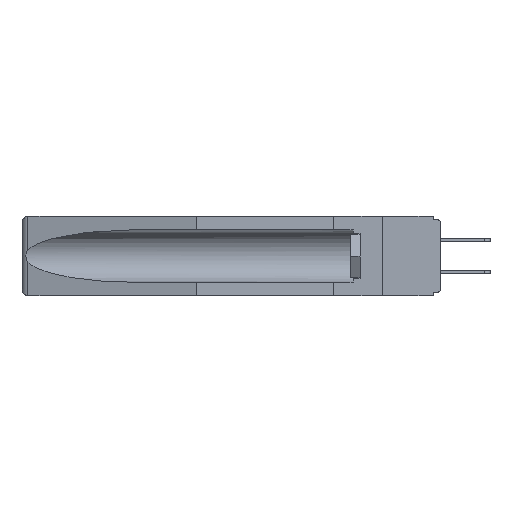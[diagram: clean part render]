
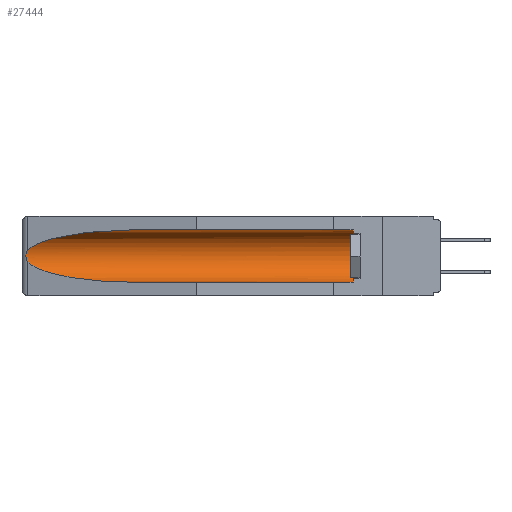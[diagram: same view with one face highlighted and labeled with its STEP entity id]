
A CAD part, left-side view. The second image highlights one B-rep face of the part: STEP entity #27444.
In plain terms, the highlighted cylindrical face has radius 2.857 mm (diameter 5.715 mm), a partial arc.
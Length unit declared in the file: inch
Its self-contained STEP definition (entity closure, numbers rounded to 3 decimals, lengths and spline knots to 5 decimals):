
#496 = CARTESIAN_POINT ( 'NONE',  ( 0.155, 1.07973, -0.059 ) ) ;
#643 = ORIENTED_EDGE ( 'NONE', *, *, #29345, .T. ) ;
#937 = CARTESIAN_POINT ( 'NONE',  ( 0.155, 1.07973, -0.284 ) ) ;
#1045 = CARTESIAN_POINT ( 'NONE',  ( 0.2675, 1.53308, -0.17534 ) ) ;
#1240 = CARTESIAN_POINT ( 'NONE',  ( 0.21114, 1.30732, -0.284 ) ) ;
#2816 = ORIENTED_EDGE ( 'NONE', *, *, #14359, .T. ) ;
#3269 = LINE ( 'NONE', #20191, #4945 ) ;
#3373 =( BOUNDED_CURVE ( )  B_SPLINE_CURVE ( 3, ( #26966, #29349, #1240, #937 ),
 .UNSPECIFIED., .F., .F. ) 
 B_SPLINE_CURVE_WITH_KNOTS ( ( 4, 4 ),
 ( 0.1948, 1.5708 ),
 .UNSPECIFIED. ) 
 CURVE ( )  GEOMETRIC_REPRESENTATION_ITEM ( )  RATIONAL_B_SPLINE_CURVE ( ( 1., 0.848, 0.848, 1. ) ) 
 REPRESENTATION_ITEM ( '' )  );
#3856 = DIRECTION ( 'NONE',  ( 0., 1., 0. ) ) ;
#4360 = CARTESIAN_POINT ( 'NONE',  ( 0.155, 0.126, -0.284 ) ) ;
#4464 = VERTEX_POINT ( 'NONE', #4360 ) ;
#4945 = VECTOR ( 'NONE', #3856, 39.37008 ) ;
#5256 = B_SPLINE_CURVE_WITH_KNOTS ( 'NONE', 3,
 ( #29054, #17379, #21716, #12756, #12349, #1045, #10107, #22134, #5476, #19750 ),
 .UNSPECIFIED., .F., .F.,
 ( 4, 2, 2, 2, 4 ),
 ( 0., 0.00029, 0.00058, 0.00087, 0.00117 ),
 .UNSPECIFIED. ) ;
#5476 = CARTESIAN_POINT ( 'NONE',  ( 0.26597, 1.5296, -0.19026 ) ) ;
#5638 = ORIENTED_EDGE ( 'NONE', *, *, #29744, .T. ) ;
#6762 = CARTESIAN_POINT ( 'NONE',  ( 0.155, 1.07973, -0.284 ) ) ;
#7711 = FACE_OUTER_BOUND ( 'NONE', #21540, .T. ) ;
#7997 = CARTESIAN_POINT ( 'NONE',  ( 0.155, 1.07973, -0.059 ) ) ;
#8139 = DIRECTION ( 'NONE',  ( 0., 1., 0. ) ) ;
#8289 = CARTESIAN_POINT ( 'NONE',  ( 0.26537, 1.52718, -0.14972 ) ) ;
#8427 = VECTOR ( 'NONE', #8139, 39.37008 ) ;
#10078 = DIRECTION ( 'NONE',  ( 0., 0., 1. ) ) ;
#10107 = CARTESIAN_POINT ( 'NONE',  ( 0.2673, 1.53269, -0.17917 ) ) ;
#10977 = CYLINDRICAL_SURFACE ( 'NONE', #28763, 0.1125 ) ;
#12308 = EDGE_CURVE ( 'NONE', #12844, #26190, #5256, .T. ) ;
#12349 = CARTESIAN_POINT ( 'NONE',  ( 0.2675, 1.53308, -0.16763 ) ) ;
#12756 = CARTESIAN_POINT ( 'NONE',  ( 0.2673, 1.5327, -0.16383 ) ) ;
#12844 = VERTEX_POINT ( 'NONE', #15924 ) ;
#13463 = DIRECTION ( 'NONE',  ( 0., -1., 0. ) ) ;
#14108 = CIRCLE ( 'NONE', #27047, 0.1125 ) ;
#14334 = VERTEX_POINT ( 'NONE', #17928 ) ;
#14359 = EDGE_CURVE ( 'NONE', #14334, #29452, #3269, .T. ) ;
#14971 = CARTESIAN_POINT ( 'NONE',  ( 0.155, -0.30754, -0.284 ) ) ;
#15711 = EDGE_CURVE ( 'NONE', #4464, #17910, #28707, .T. ) ;
#15924 = CARTESIAN_POINT ( 'NONE',  ( 0.26537, 1.52718, -0.14972 ) ) ;
#17042 = DIRECTION ( 'NONE',  ( 0., 1., 0. ) ) ;
#17379 = CARTESIAN_POINT ( 'NONE',  ( 0.26597, 1.52961, -0.15275 ) ) ;
#17608 = CARTESIAN_POINT ( 'NONE',  ( 0.25451, 1.48313, -0.09465 ) ) ;
#17910 = VERTEX_POINT ( 'NONE', #6762 ) ;
#17928 = CARTESIAN_POINT ( 'NONE',  ( 0.155, 0.126, -0.059 ) ) ;
#18120 = DIRECTION ( 'NONE',  ( 0., 0., 1. ) ) ;
#18223 = CARTESIAN_POINT ( 'NONE',  ( 0.155, 0.126, -0.1715 ) ) ;
#19185 = ORIENTED_EDGE ( 'NONE', *, *, #15711, .F. ) ;
#19750 = CARTESIAN_POINT ( 'NONE',  ( 0.26537, 1.52718, -0.19328 ) ) ;
#20191 = CARTESIAN_POINT ( 'NONE',  ( 0.155, -0.30754, -0.059 ) ) ;
#21540 = EDGE_LOOP ( 'NONE', ( #29189, #26014, #643, #19185, #5638, #2816 ) ) ;
#21716 = CARTESIAN_POINT ( 'NONE',  ( 0.26654, 1.53092, -0.15636 ) ) ;
#22134 = CARTESIAN_POINT ( 'NONE',  ( 0.26655, 1.53094, -0.18657 ) ) ;
#22245 = CARTESIAN_POINT ( 'NONE',  ( 0.26537, 1.52718, -0.19328 ) ) ;
#24445 = CARTESIAN_POINT ( 'NONE',  ( 0.21114, 1.30732, -0.059 ) ) ;
#24864 =( BOUNDED_CURVE ( )  B_SPLINE_CURVE ( 3, ( #7997, #24445, #17608, #8289 ),
 .UNSPECIFIED., .F., .F. ) 
 B_SPLINE_CURVE_WITH_KNOTS ( ( 4, 4 ),
 ( 4.71239, 6.08839 ),
 .UNSPECIFIED. ) 
 CURVE ( )  GEOMETRIC_REPRESENTATION_ITEM ( )  RATIONAL_B_SPLINE_CURVE ( ( 1., 0.848, 0.848, 1. ) ) 
 REPRESENTATION_ITEM ( '' )  );
#26014 = ORIENTED_EDGE ( 'NONE', *, *, #12308, .T. ) ;
#26190 = VERTEX_POINT ( 'NONE', #22245 ) ;
#26966 = CARTESIAN_POINT ( 'NONE',  ( 0.26537, 1.52718, -0.19328 ) ) ;
#27047 = AXIS2_PLACEMENT_3D ( 'NONE', #18223, #13463, #18120 ) ;
#27444 = ADVANCED_FACE ( 'NONE', ( #7711 ), #10977, .F. ) ;
#27722 = EDGE_CURVE ( 'NONE', #29452, #12844, #24864, .T. ) ;
#28707 = LINE ( 'NONE', #14971, #8427 ) ;
#28763 = AXIS2_PLACEMENT_3D ( 'NONE', #29243, #17042, #10078 ) ;
#29054 = CARTESIAN_POINT ( 'NONE',  ( 0.26537, 1.52718, -0.14972 ) ) ;
#29189 = ORIENTED_EDGE ( 'NONE', *, *, #27722, .T. ) ;
#29243 = CARTESIAN_POINT ( 'NONE',  ( 0.155, -0.30754, -0.1715 ) ) ;
#29345 = EDGE_CURVE ( 'NONE', #26190, #17910, #3373, .T. ) ;
#29349 = CARTESIAN_POINT ( 'NONE',  ( 0.25451, 1.48313, -0.24835 ) ) ;
#29452 = VERTEX_POINT ( 'NONE', #496 ) ;
#29744 = EDGE_CURVE ( 'NONE', #4464, #14334, #14108, .T. ) ;
